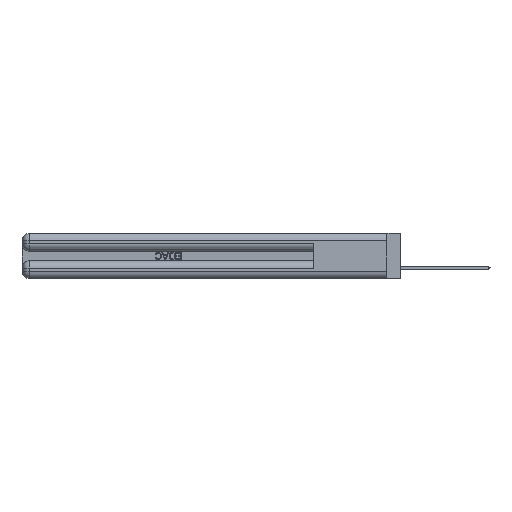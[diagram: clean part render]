
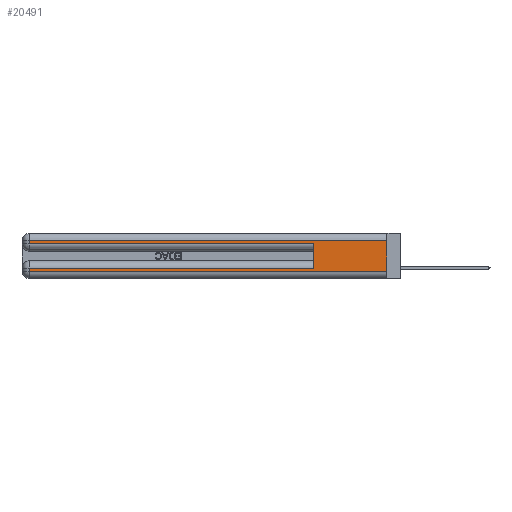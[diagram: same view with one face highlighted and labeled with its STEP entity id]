
A CAD part, left-side view. The second image highlights one B-rep face of the part: STEP entity #20491.
In plain terms, the highlighted planar face has unit normal (-1, 0, 0).
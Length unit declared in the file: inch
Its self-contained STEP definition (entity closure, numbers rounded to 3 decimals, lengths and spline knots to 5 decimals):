
#1311 = EDGE_CURVE ( 'NONE', #10935, #25554, #27772, .T. ) ;
#1429 = VECTOR ( 'NONE', #35923, 39.37008 ) ;
#1452 = CARTESIAN_POINT ( 'NONE',  ( 0., 0., 0.31 ) ) ;
#1649 = DIRECTION ( 'NONE',  ( 0., 0., -1. ) ) ;
#2763 = VECTOR ( 'NONE', #39060, 39.37008 ) ;
#2946 = CARTESIAN_POINT ( 'NONE',  ( 0., 0., 0.285 ) ) ;
#3677 = VERTEX_POINT ( 'NONE', #20366 ) ;
#4061 = VERTEX_POINT ( 'NONE', #1452 ) ;
#4115 = VECTOR ( 'NONE', #1649, 39.37008 ) ;
#4303 = CARTESIAN_POINT ( 'NONE',  ( 0., 0., 0.37 ) ) ;
#5036 = VECTOR ( 'NONE', #25142, 39.37008 ) ;
#5851 = DIRECTION ( 'NONE',  ( 0., 0., -1. ) ) ;
#5856 = EDGE_CURVE ( 'NONE', #32361, #10935, #33634, .T. ) ;
#5912 = VERTEX_POINT ( 'NONE', #29594 ) ;
#5927 = DIRECTION ( 'NONE',  ( 0., 1., 0. ) ) ;
#6015 = ORIENTED_EDGE ( 'NONE', *, *, #25098, .T. ) ;
#6873 = DIRECTION ( 'NONE',  ( 0., 0., -1. ) ) ;
#7205 = CARTESIAN_POINT ( 'NONE',  ( 0., 2.94, 0.37 ) ) ;
#7461 = LINE ( 'NONE', #23723, #35541 ) ;
#9254 = VECTOR ( 'NONE', #5927, 39.37008 ) ;
#9775 = DIRECTION ( 'NONE',  ( 1., 0., 0. ) ) ;
#10554 = ORIENTED_EDGE ( 'NONE', *, *, #5856, .T. ) ;
#10935 = VERTEX_POINT ( 'NONE', #39727 ) ;
#11084 = CARTESIAN_POINT ( 'NONE',  ( 0., 2.94, 0.06 ) ) ;
#13700 = PLANE ( 'NONE',  #49791 ) ;
#14502 = EDGE_LOOP ( 'NONE', ( #31712, #28470, #44695, #6015, #29277, #10554, #17681, #23802 ) ) ;
#14710 = CARTESIAN_POINT ( 'NONE',  ( 0., 0., 0.06 ) ) ;
#17681 = ORIENTED_EDGE ( 'NONE', *, *, #1311, .T. ) ;
#18529 = CARTESIAN_POINT ( 'NONE',  ( 0., 0.6, 0.145 ) ) ;
#18670 = EDGE_CURVE ( 'NONE', #32361, #48935, #44269, .T. ) ;
#20366 = CARTESIAN_POINT ( 'NONE',  ( 0., 2.94, 0.31 ) ) ;
#20491 = ADVANCED_FACE ( 'NONE', ( #26437 ), #13700, .F. ) ;
#21795 = EDGE_CURVE ( 'NONE', #4061, #3677, #47061, .T. ) ;
#23723 = CARTESIAN_POINT ( 'NONE',  ( 0., 0., 0.06 ) ) ;
#23802 = ORIENTED_EDGE ( 'NONE', *, *, #28488, .T. ) ;
#24802 = LINE ( 'NONE', #29395, #4115 ) ;
#25072 = VERTEX_POINT ( 'NONE', #14710 ) ;
#25098 = EDGE_CURVE ( 'NONE', #5912, #48935, #49717, .T. ) ;
#25142 = DIRECTION ( 'NONE',  ( 0., 1., 0. ) ) ;
#25170 = LINE ( 'NONE', #4303, #1429 ) ;
#25554 = VERTEX_POINT ( 'NONE', #11084 ) ;
#26437 = FACE_OUTER_BOUND ( 'NONE', #14502, .T. ) ;
#27069 = EDGE_CURVE ( 'NONE', #4061, #25072, #25170, .T. ) ;
#27772 = LINE ( 'NONE', #7205, #49074 ) ;
#28470 = ORIENTED_EDGE ( 'NONE', *, *, #21795, .T. ) ;
#28488 = EDGE_CURVE ( 'NONE', #25554, #25072, #7461, .T. ) ;
#29277 = ORIENTED_EDGE ( 'NONE', *, *, #18670, .F. ) ;
#29395 = CARTESIAN_POINT ( 'NONE',  ( 0., 2.94, 0.37 ) ) ;
#29594 = CARTESIAN_POINT ( 'NONE',  ( 0., 2.94, 0.285 ) ) ;
#30270 = DIRECTION ( 'NONE',  ( 0., 0., 1. ) ) ;
#31712 = ORIENTED_EDGE ( 'NONE', *, *, #27069, .F. ) ;
#32361 = VERTEX_POINT ( 'NONE', #41691 ) ;
#32804 = CARTESIAN_POINT ( 'NONE',  ( 0., 0., 0.31 ) ) ;
#33634 = LINE ( 'NONE', #48844, #9254 ) ;
#33752 = CARTESIAN_POINT ( 'NONE',  ( 0., 0., 0.37 ) ) ;
#35541 = VECTOR ( 'NONE', #47417, 39.37008 ) ;
#35923 = DIRECTION ( 'NONE',  ( 0., 0., -1. ) ) ;
#36582 = CARTESIAN_POINT ( 'NONE',  ( 0., 0.6, 0.285 ) ) ;
#39060 = DIRECTION ( 'NONE',  ( 0., -1., 0. ) ) ;
#39727 = CARTESIAN_POINT ( 'NONE',  ( 0., 2.94, 0.085 ) ) ;
#41691 = CARTESIAN_POINT ( 'NONE',  ( 0., 0.6, 0.085 ) ) ;
#43806 = EDGE_CURVE ( 'NONE', #3677, #5912, #24802, .T. ) ;
#44269 = LINE ( 'NONE', #18529, #45473 ) ;
#44695 = ORIENTED_EDGE ( 'NONE', *, *, #43806, .T. ) ;
#45473 = VECTOR ( 'NONE', #30270, 39.37008 ) ;
#47061 = LINE ( 'NONE', #32804, #5036 ) ;
#47417 = DIRECTION ( 'NONE',  ( 0., -1., 0. ) ) ;
#48844 = CARTESIAN_POINT ( 'NONE',  ( 0., 0., 0.085 ) ) ;
#48935 = VERTEX_POINT ( 'NONE', #36582 ) ;
#49074 = VECTOR ( 'NONE', #6873, 39.37008 ) ;
#49717 = LINE ( 'NONE', #2946, #2763 ) ;
#49791 = AXIS2_PLACEMENT_3D ( 'NONE', #33752, #9775, #5851 ) ;
